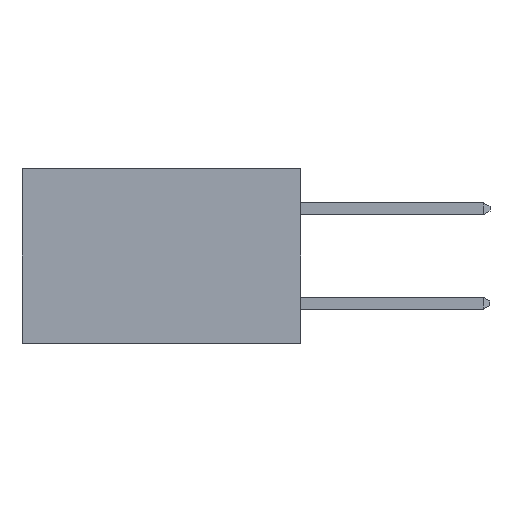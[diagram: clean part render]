
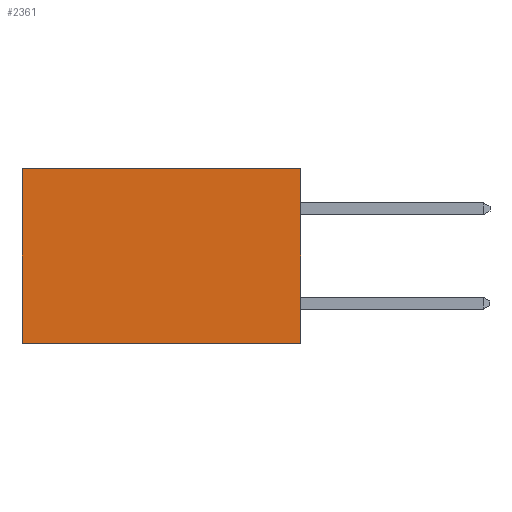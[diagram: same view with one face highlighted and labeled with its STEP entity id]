
A CAD part, left-side view. The second image highlights one B-rep face of the part: STEP entity #2361.
In plain terms, the highlighted planar face has unit normal (-1, 0, 0).
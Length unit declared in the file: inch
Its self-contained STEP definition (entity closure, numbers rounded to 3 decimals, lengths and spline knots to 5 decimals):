
#106 = CARTESIAN_POINT ( 'NONE',  ( 0.277, 0.59, 0. ) ) ;
#265 = DIRECTION ( 'NONE',  ( 0., 0., -1. ) ) ;
#303 = CARTESIAN_POINT ( 'NONE',  ( 0.277, 0.59, -0.37 ) ) ;
#801 = VECTOR ( 'NONE', #3701, 39.37008 ) ;
#1033 = DIRECTION ( 'NONE',  ( 0., 1., 0. ) ) ;
#1053 = CARTESIAN_POINT ( 'NONE',  ( 0.277, 0., 0. ) ) ;
#1084 = EDGE_CURVE ( 'NONE', #6774, #6048, #4860, .T. ) ;
#1259 = EDGE_CURVE ( 'NONE', #6218, #6048, #4216, .T. ) ;
#1298 = EDGE_CURVE ( 'NONE', #6423, #6218, #3790, .T. ) ;
#1303 = VECTOR ( 'NONE', #265, 39.37008 ) ;
#1720 = PLANE ( 'NONE',  #3199 ) ;
#2035 = ORIENTED_EDGE ( 'NONE', *, *, #1084, .T. ) ;
#2095 = EDGE_LOOP ( 'NONE', ( #2035, #5803, #6036, #5760 ) ) ;
#2361 = ADVANCED_FACE ( 'NONE', ( #3479 ), #1720, .F. ) ;
#2456 = CARTESIAN_POINT ( 'NONE',  ( 0.277, 0.59, -0.37 ) ) ;
#3102 = VECTOR ( 'NONE', #1033, 39.37008 ) ;
#3199 = AXIS2_PLACEMENT_3D ( 'NONE', #4875, #3912, #3814 ) ;
#3479 = FACE_OUTER_BOUND ( 'NONE', #2095, .T. ) ;
#3701 = DIRECTION ( 'NONE',  ( 0., 1., 0. ) ) ;
#3790 = LINE ( 'NONE', #7313, #6846 ) ;
#3814 = DIRECTION ( 'NONE',  ( 0., 0., -1. ) ) ;
#3912 = DIRECTION ( 'NONE',  ( 1., 0., 0. ) ) ;
#3927 = CARTESIAN_POINT ( 'NONE',  ( 0.277, 0., 0. ) ) ;
#4216 = LINE ( 'NONE', #5758, #801 ) ;
#4860 = LINE ( 'NONE', #2456, #1303 ) ;
#4875 = CARTESIAN_POINT ( 'NONE',  ( 0.277, 0., -0.37 ) ) ;
#5575 = EDGE_CURVE ( 'NONE', #6423, #6774, #7885, .T. ) ;
#5587 = DIRECTION ( 'NONE',  ( 0., 0., -1. ) ) ;
#5758 = CARTESIAN_POINT ( 'NONE',  ( 0.277, 0., -0.37 ) ) ;
#5760 = ORIENTED_EDGE ( 'NONE', *, *, #5575, .T. ) ;
#5803 = ORIENTED_EDGE ( 'NONE', *, *, #1259, .F. ) ;
#5859 = CARTESIAN_POINT ( 'NONE',  ( 0.277, 0., -0.37 ) ) ;
#6036 = ORIENTED_EDGE ( 'NONE', *, *, #1298, .F. ) ;
#6048 = VERTEX_POINT ( 'NONE', #303 ) ;
#6218 = VERTEX_POINT ( 'NONE', #5859 ) ;
#6423 = VERTEX_POINT ( 'NONE', #3927 ) ;
#6774 = VERTEX_POINT ( 'NONE', #106 ) ;
#6846 = VECTOR ( 'NONE', #5587, 39.37008 ) ;
#7313 = CARTESIAN_POINT ( 'NONE',  ( 0.277, 0., -0.37 ) ) ;
#7885 = LINE ( 'NONE', #1053, #3102 ) ;
